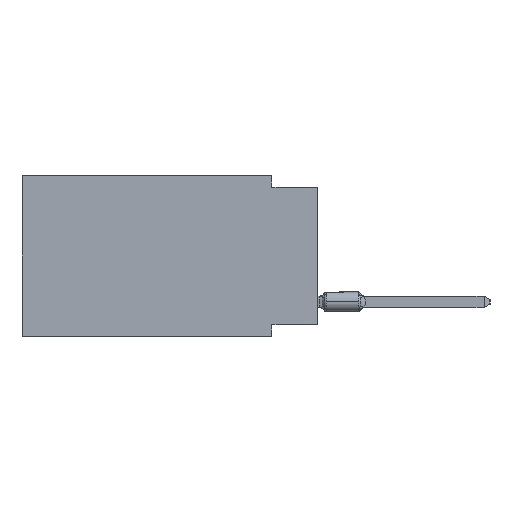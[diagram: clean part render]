
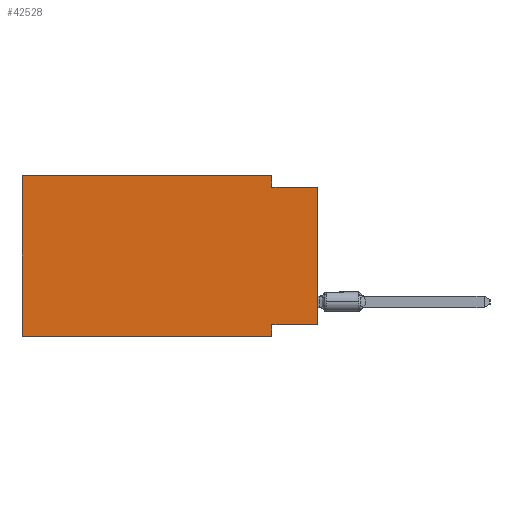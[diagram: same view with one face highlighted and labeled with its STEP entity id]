
A CAD part, left-side view. The second image highlights one B-rep face of the part: STEP entity #42528.
In plain terms, the highlighted planar face has unit normal (-1, 0, 0).
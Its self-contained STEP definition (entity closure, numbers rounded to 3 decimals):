
#701 = VERTEX_POINT ( 'NONE', #30380 ) ;
#1531 = ORIENTED_EDGE ( 'NONE', *, *, #44943, .F. ) ;
#5200 = DIRECTION ( 'NONE',  ( 0., -1., 0. ) ) ;
#6738 = VECTOR ( 'NONE', #21648, 1000. ) ;
#7308 = VECTOR ( 'NONE', #33467, 1000. ) ;
#7562 = CARTESIAN_POINT ( 'NONE',  ( 0., 2.54, -8.255 ) ) ;
#7628 = EDGE_CURVE ( 'NONE', #12272, #14859, #23866, .T. ) ;
#7752 = LINE ( 'NONE', #18814, #7308 ) ;
#8641 = DIRECTION ( 'NONE',  ( 1., 0., 0. ) ) ;
#10377 = ORIENTED_EDGE ( 'NONE', *, *, #20615, .T. ) ;
#12179 = CARTESIAN_POINT ( 'NONE',  ( 0., 16.383, 0. ) ) ;
#12272 = VERTEX_POINT ( 'NONE', #16981 ) ;
#12758 = VERTEX_POINT ( 'NONE', #12799 ) ;
#12799 = CARTESIAN_POINT ( 'NONE',  ( 0., 2.54, -8.89 ) ) ;
#13674 = LINE ( 'NONE', #20674, #39574 ) ;
#14305 = EDGE_CURVE ( 'NONE', #38961, #12758, #40908, .T. ) ;
#14859 = VERTEX_POINT ( 'NONE', #32872 ) ;
#14968 = EDGE_CURVE ( 'NONE', #14859, #701, #23490, .T. ) ;
#15160 = CARTESIAN_POINT ( 'NONE',  ( 0., 0., 0. ) ) ;
#15235 = CARTESIAN_POINT ( 'NONE',  ( 0., 2.54, 0. ) ) ;
#15642 = PLANE ( 'NONE',  #38859 ) ;
#15706 = DIRECTION ( 'NONE',  ( 0., 0., -1. ) ) ;
#15756 = EDGE_CURVE ( 'NONE', #46296, #43227, #7752, .T. ) ;
#16981 = CARTESIAN_POINT ( 'NONE',  ( 0., 16.383, -8.89 ) ) ;
#18814 = CARTESIAN_POINT ( 'NONE',  ( 0., 0., -0.635 ) ) ;
#19538 = VECTOR ( 'NONE', #5200, 1000. ) ;
#19910 = LINE ( 'NONE', #30949, #29993 ) ;
#20241 = DIRECTION ( 'NONE',  ( 0., 0., 1. ) ) ;
#20615 = EDGE_CURVE ( 'NONE', #24813, #43227, #25978, .T. ) ;
#20674 = CARTESIAN_POINT ( 'NONE',  ( 0., 0., -8.255 ) ) ;
#21648 = DIRECTION ( 'NONE',  ( 0., 0., 1. ) ) ;
#22707 = VECTOR ( 'NONE', #15706, 1000. ) ;
#22921 = LINE ( 'NONE', #15235, #22707 ) ;
#23490 = LINE ( 'NONE', #12179, #19538 ) ;
#23813 = CARTESIAN_POINT ( 'NONE',  ( 0., 16.383, 0. ) ) ;
#23866 = LINE ( 'NONE', #42317, #35290 ) ;
#24813 = VERTEX_POINT ( 'NONE', #27897 ) ;
#24921 = DIRECTION ( 'NONE',  ( 0., -1., 0. ) ) ;
#25978 = LINE ( 'NONE', #15160, #6738 ) ;
#27380 = ORIENTED_EDGE ( 'NONE', *, *, #14305, .F. ) ;
#27897 = CARTESIAN_POINT ( 'NONE',  ( 0., 0., -8.255 ) ) ;
#28350 = DIRECTION ( 'NONE',  ( 0., 1., 0. ) ) ;
#29993 = VECTOR ( 'NONE', #24921, 1000. ) ;
#30125 = DIRECTION ( 'NONE',  ( 0., 0., -1. ) ) ;
#30380 = CARTESIAN_POINT ( 'NONE',  ( 0., 2.54, 0. ) ) ;
#30605 = CARTESIAN_POINT ( 'NONE',  ( 0., 2.54, -8.89 ) ) ;
#30766 = FACE_OUTER_BOUND ( 'NONE', #47503, .T. ) ;
#30949 = CARTESIAN_POINT ( 'NONE',  ( 0., 16.383, -8.89 ) ) ;
#32872 = CARTESIAN_POINT ( 'NONE',  ( 0., 16.383, 0. ) ) ;
#33467 = DIRECTION ( 'NONE',  ( 0., -1., 0. ) ) ;
#33869 = ORIENTED_EDGE ( 'NONE', *, *, #14968, .F. ) ;
#35290 = VECTOR ( 'NONE', #20241, 1000. ) ;
#36813 = EDGE_CURVE ( 'NONE', #12272, #12758, #19910, .T. ) ;
#38859 = AXIS2_PLACEMENT_3D ( 'NONE', #23813, #8641, #45627 ) ;
#38961 = VERTEX_POINT ( 'NONE', #7562 ) ;
#39574 = VECTOR ( 'NONE', #28350, 1000. ) ;
#40908 = LINE ( 'NONE', #30605, #40938 ) ;
#40938 = VECTOR ( 'NONE', #30125, 1000. ) ;
#41970 = CARTESIAN_POINT ( 'NONE',  ( 0., 0., -0.635 ) ) ;
#42317 = CARTESIAN_POINT ( 'NONE',  ( 0., 16.383, 0. ) ) ;
#42528 = ADVANCED_FACE ( 'NONE', ( #30766 ), #15642, .F. ) ;
#42870 = ORIENTED_EDGE ( 'NONE', *, *, #7628, .F. ) ;
#43106 = ORIENTED_EDGE ( 'NONE', *, *, #44386, .F. ) ;
#43227 = VERTEX_POINT ( 'NONE', #41970 ) ;
#44386 = EDGE_CURVE ( 'NONE', #701, #46296, #22921, .T. ) ;
#44679 = ORIENTED_EDGE ( 'NONE', *, *, #15756, .F. ) ;
#44943 = EDGE_CURVE ( 'NONE', #24813, #38961, #13674, .T. ) ;
#45627 = DIRECTION ( 'NONE',  ( 0., 0., -1. ) ) ;
#45996 = ORIENTED_EDGE ( 'NONE', *, *, #36813, .T. ) ;
#46296 = VERTEX_POINT ( 'NONE', #46538 ) ;
#46538 = CARTESIAN_POINT ( 'NONE',  ( 0., 2.54, -0.635 ) ) ;
#47503 = EDGE_LOOP ( 'NONE', ( #10377, #44679, #43106, #33869, #42870, #45996, #27380, #1531 ) ) ;
